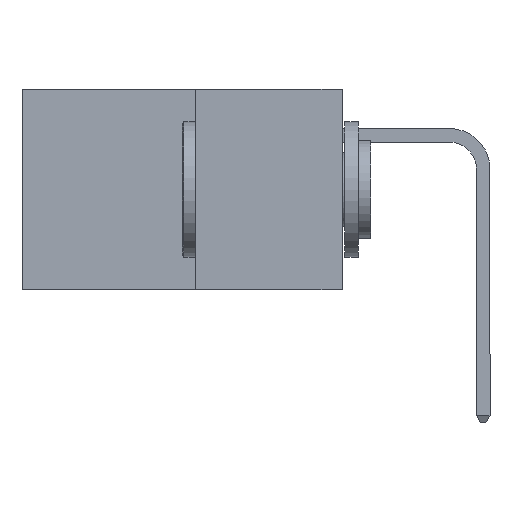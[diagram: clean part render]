
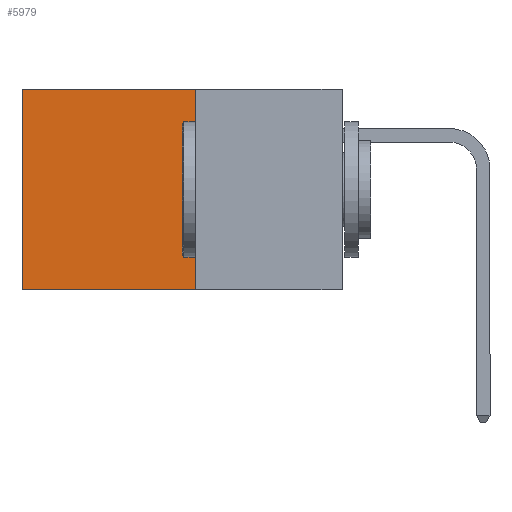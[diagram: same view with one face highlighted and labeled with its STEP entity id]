
A CAD part, left-side view. The second image highlights one B-rep face of the part: STEP entity #5979.
In plain terms, the highlighted planar face has unit normal (-1, 0, 0).
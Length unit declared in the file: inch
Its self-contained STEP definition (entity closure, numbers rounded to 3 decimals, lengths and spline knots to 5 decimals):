
#101 = VECTOR ( 'NONE', #8459, 39.37008 ) ;
#715 = ORIENTED_EDGE ( 'NONE', *, *, #1788, .T. ) ;
#903 = CARTESIAN_POINT ( 'NONE',  ( 0.277, 0.59, -0.37 ) ) ;
#1788 = EDGE_CURVE ( 'NONE', #2766, #2372, #18288, .T. ) ;
#1946 = CARTESIAN_POINT ( 'NONE',  ( 0.277, 0.27, -0.37 ) ) ;
#2372 = VERTEX_POINT ( 'NONE', #16597 ) ;
#2766 = VERTEX_POINT ( 'NONE', #14598 ) ;
#4389 = LINE ( 'NONE', #10883, #21701 ) ;
#4494 = CARTESIAN_POINT ( 'NONE',  ( 0.277, 0.59, -0.37 ) ) ;
#5979 = ADVANCED_FACE ( 'NONE', ( #19061 ), #21714, .F. ) ;
#7060 = VECTOR ( 'NONE', #18963, 39.37008 ) ;
#7334 = VERTEX_POINT ( 'NONE', #4494 ) ;
#8455 = CARTESIAN_POINT ( 'NONE',  ( 0.277, 0.27, 0. ) ) ;
#8459 = DIRECTION ( 'NONE',  ( 0., 1., 0. ) ) ;
#8950 = EDGE_CURVE ( 'NONE', #21394, #7334, #11576, .T. ) ;
#9096 = EDGE_CURVE ( 'NONE', #2766, #21394, #4389, .T. ) ;
#10883 = CARTESIAN_POINT ( 'NONE',  ( 0.277, 0.27, -0.37 ) ) ;
#11293 = AXIS2_PLACEMENT_3D ( 'NONE', #21586, #21013, #20821 ) ;
#11576 = LINE ( 'NONE', #1946, #7060 ) ;
#11778 = EDGE_CURVE ( 'NONE', #2372, #7334, #13374, .T. ) ;
#12285 = CARTESIAN_POINT ( 'NONE',  ( 0.277, 0.27, -0.37 ) ) ;
#12605 = DIRECTION ( 'NONE',  ( 0., 0., -1. ) ) ;
#13374 = LINE ( 'NONE', #903, #21657 ) ;
#13550 = ORIENTED_EDGE ( 'NONE', *, *, #11778, .T. ) ;
#14598 = CARTESIAN_POINT ( 'NONE',  ( 0.277, 0.27, 0. ) ) ;
#16597 = CARTESIAN_POINT ( 'NONE',  ( 0.277, 0.59, 0. ) ) ;
#17914 = DIRECTION ( 'NONE',  ( 0., 0., -1. ) ) ;
#18288 = LINE ( 'NONE', #8455, #101 ) ;
#18963 = DIRECTION ( 'NONE',  ( 0., 1., 0. ) ) ;
#19061 = FACE_OUTER_BOUND ( 'NONE', #20000, .T. ) ;
#19729 = ORIENTED_EDGE ( 'NONE', *, *, #9096, .F. ) ;
#20000 = EDGE_LOOP ( 'NONE', ( #13550, #21382, #19729, #715 ) ) ;
#20821 = DIRECTION ( 'NONE',  ( 0., 0., -1. ) ) ;
#21013 = DIRECTION ( 'NONE',  ( 1., 0., 0. ) ) ;
#21382 = ORIENTED_EDGE ( 'NONE', *, *, #8950, .F. ) ;
#21394 = VERTEX_POINT ( 'NONE', #12285 ) ;
#21586 = CARTESIAN_POINT ( 'NONE',  ( 0.277, 0.27, -0.37 ) ) ;
#21657 = VECTOR ( 'NONE', #17914, 39.37008 ) ;
#21701 = VECTOR ( 'NONE', #12605, 39.37008 ) ;
#21714 = PLANE ( 'NONE',  #11293 ) ;
